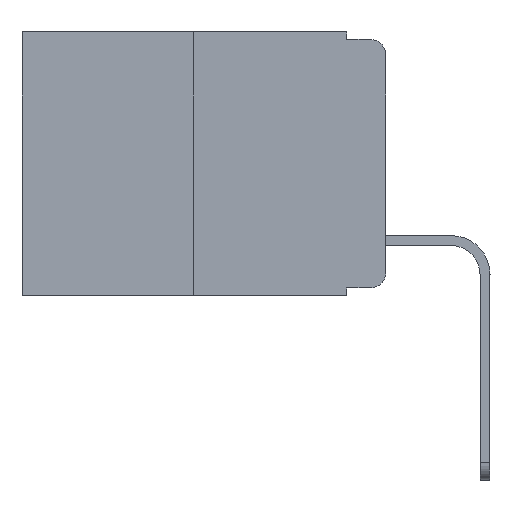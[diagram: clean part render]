
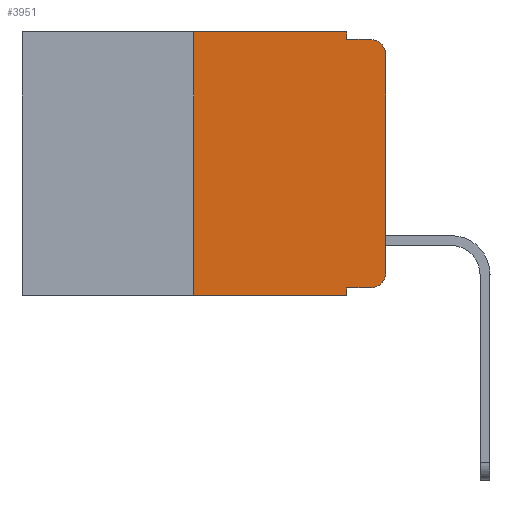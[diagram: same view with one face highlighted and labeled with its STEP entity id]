
A CAD part, left-side view. The second image highlights one B-rep face of the part: STEP entity #3951.
In plain terms, the highlighted planar face has unit normal (-1, 0, 0).
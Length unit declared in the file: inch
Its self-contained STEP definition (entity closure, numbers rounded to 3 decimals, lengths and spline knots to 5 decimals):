
#174 = VECTOR ( 'NONE', #3355, 39.37008 ) ;
#323 = DIRECTION ( 'NONE',  ( -1., 0., 0. ) ) ;
#488 = ORIENTED_EDGE ( 'NONE', *, *, #8297, .T. ) ;
#958 = LINE ( 'NONE', #17991, #15737 ) ;
#1249 = ORIENTED_EDGE ( 'NONE', *, *, #10036, .T. ) ;
#1389 = AXIS2_PLACEMENT_3D ( 'NONE', #17599, #11719, #11835 ) ;
#1697 = EDGE_CURVE ( 'NONE', #3849, #6895, #4745, .T. ) ;
#1803 = PLANE ( 'NONE',  #10446 ) ;
#1987 = ORIENTED_EDGE ( 'NONE', *, *, #7157, .T. ) ;
#1989 = DIRECTION ( 'NONE',  ( 1., 0., 0. ) ) ;
#2281 = CARTESIAN_POINT ( 'NONE',  ( 0., 0.051, -0.01 ) ) ;
#2936 = EDGE_CURVE ( 'NONE', #3849, #6368, #5798, .T. ) ;
#3190 = CARTESIAN_POINT ( 'NONE',  ( 0., 0., -0.313 ) ) ;
#3355 = DIRECTION ( 'NONE',  ( 0., 0., 1. ) ) ;
#3689 = DIRECTION ( 'NONE',  ( 0., -1., 0. ) ) ;
#3849 = VERTEX_POINT ( 'NONE', #12003 ) ;
#3951 = ADVANCED_FACE ( 'NONE', ( #13840 ), #1803, .F. ) ;
#4141 = ORIENTED_EDGE ( 'NONE', *, *, #15373, .T. ) ;
#4556 = CARTESIAN_POINT ( 'NONE',  ( 0., 0.02, -0.03 ) ) ;
#4678 = ORIENTED_EDGE ( 'NONE', *, *, #4796, .F. ) ;
#4745 = LINE ( 'NONE', #18502, #13244 ) ;
#4796 = EDGE_CURVE ( 'NONE', #5421, #17242, #11567, .T. ) ;
#4831 = CARTESIAN_POINT ( 'NONE',  ( 0., 0.473, 0. ) ) ;
#4922 = LINE ( 'NONE', #2281, #6964 ) ;
#4992 = CARTESIAN_POINT ( 'NONE',  ( 0., 0.473, 0. ) ) ;
#5192 = CARTESIAN_POINT ( 'NONE',  ( 0., 0.051, -0.333 ) ) ;
#5421 = VERTEX_POINT ( 'NONE', #10414 ) ;
#5792 = CARTESIAN_POINT ( 'NONE',  ( 0., 0.051, -0.01 ) ) ;
#5798 = LINE ( 'NONE', #5192, #17212 ) ;
#5869 = ORIENTED_EDGE ( 'NONE', *, *, #9494, .F. ) ;
#5936 = CARTESIAN_POINT ( 'NONE',  ( 0., 0., -0.03 ) ) ;
#6339 = ORIENTED_EDGE ( 'NONE', *, *, #2936, .T. ) ;
#6368 = VERTEX_POINT ( 'NONE', #15723 ) ;
#6520 = CARTESIAN_POINT ( 'NONE',  ( 0., 0.25, -0.343 ) ) ;
#6633 = CIRCLE ( 'NONE', #1389, 0.02 ) ;
#6726 = ORIENTED_EDGE ( 'NONE', *, *, #1697, .F. ) ;
#6820 = LINE ( 'NONE', #16221, #17983 ) ;
#6895 = VERTEX_POINT ( 'NONE', #13514 ) ;
#6964 = VECTOR ( 'NONE', #13563, 39.37008 ) ;
#7157 = EDGE_CURVE ( 'NONE', #9408, #17945, #9501, .T. ) ;
#7344 = DIRECTION ( 'NONE',  ( 0., 0., -1. ) ) ;
#7728 = DIRECTION ( 'NONE',  ( 0., 0., -1. ) ) ;
#7731 = CARTESIAN_POINT ( 'NONE',  ( 0., 0.02, -0.01 ) ) ;
#7856 = EDGE_LOOP ( 'NONE', ( #4141, #1987, #10000, #14556, #4678, #5869, #488, #6726, #6339, #1249 ) ) ;
#8297 = EDGE_CURVE ( 'NONE', #9057, #6895, #13403, .T. ) ;
#9057 = VERTEX_POINT ( 'NONE', #6520 ) ;
#9408 = VERTEX_POINT ( 'NONE', #5936 ) ;
#9482 = DIRECTION ( 'NONE',  ( 0., 0., -1. ) ) ;
#9494 = EDGE_CURVE ( 'NONE', #9057, #5421, #16267, .T. ) ;
#9501 = CIRCLE ( 'NONE', #12022, 0.02 ) ;
#10000 = ORIENTED_EDGE ( 'NONE', *, *, #13081, .F. ) ;
#10036 = EDGE_CURVE ( 'NONE', #6368, #13431, #6633, .T. ) ;
#10414 = CARTESIAN_POINT ( 'NONE',  ( 0., 0.25, 0. ) ) ;
#10446 = AXIS2_PLACEMENT_3D ( 'NONE', #4831, #1989, #7728 ) ;
#10905 = VECTOR ( 'NONE', #3689, 39.37008 ) ;
#11119 = DIRECTION ( 'NONE',  ( 0., -1., 0. ) ) ;
#11567 = LINE ( 'NONE', #4992, #10905 ) ;
#11719 = DIRECTION ( 'NONE',  ( -1., 0., 0. ) ) ;
#11835 = DIRECTION ( 'NONE',  ( 0., 0., -1. ) ) ;
#11914 = EDGE_CURVE ( 'NONE', #17242, #17193, #958, .T. ) ;
#12003 = CARTESIAN_POINT ( 'NONE',  ( 0., 0.051, -0.333 ) ) ;
#12022 = AXIS2_PLACEMENT_3D ( 'NONE', #4556, #323, #7344 ) ;
#12639 = DIRECTION ( 'NONE',  ( 0., 0., -1. ) ) ;
#13081 = EDGE_CURVE ( 'NONE', #17193, #17945, #4922, .T. ) ;
#13216 = CARTESIAN_POINT ( 'NONE',  ( 0., 0.473, -0.343 ) ) ;
#13244 = VECTOR ( 'NONE', #12639, 39.37008 ) ;
#13403 = LINE ( 'NONE', #13216, #14529 ) ;
#13431 = VERTEX_POINT ( 'NONE', #3190 ) ;
#13514 = CARTESIAN_POINT ( 'NONE',  ( 0., 0.051, -0.343 ) ) ;
#13563 = DIRECTION ( 'NONE',  ( 0., -1., 0. ) ) ;
#13840 = FACE_OUTER_BOUND ( 'NONE', #7856, .T. ) ;
#14529 = VECTOR ( 'NONE', #17535, 39.37008 ) ;
#14556 = ORIENTED_EDGE ( 'NONE', *, *, #11914, .F. ) ;
#14869 = CARTESIAN_POINT ( 'NONE',  ( 0., 0.25, 0. ) ) ;
#15373 = EDGE_CURVE ( 'NONE', #13431, #9408, #6820, .T. ) ;
#15723 = CARTESIAN_POINT ( 'NONE',  ( 0., 0.02, -0.333 ) ) ;
#15737 = VECTOR ( 'NONE', #9482, 39.37008 ) ;
#16221 = CARTESIAN_POINT ( 'NONE',  ( 0., 0., 0. ) ) ;
#16267 = LINE ( 'NONE', #14869, #174 ) ;
#17193 = VERTEX_POINT ( 'NONE', #5792 ) ;
#17212 = VECTOR ( 'NONE', #11119, 39.37008 ) ;
#17239 = CARTESIAN_POINT ( 'NONE',  ( 0., 0.051, 0. ) ) ;
#17242 = VERTEX_POINT ( 'NONE', #17239 ) ;
#17535 = DIRECTION ( 'NONE',  ( 0., -1., 0. ) ) ;
#17599 = CARTESIAN_POINT ( 'NONE',  ( 0., 0.02, -0.313 ) ) ;
#17644 = DIRECTION ( 'NONE',  ( 0., 0., 1. ) ) ;
#17945 = VERTEX_POINT ( 'NONE', #7731 ) ;
#17983 = VECTOR ( 'NONE', #17644, 39.37008 ) ;
#17991 = CARTESIAN_POINT ( 'NONE',  ( 0., 0.051, 0. ) ) ;
#18502 = CARTESIAN_POINT ( 'NONE',  ( 0., 0.051, 0. ) ) ;
